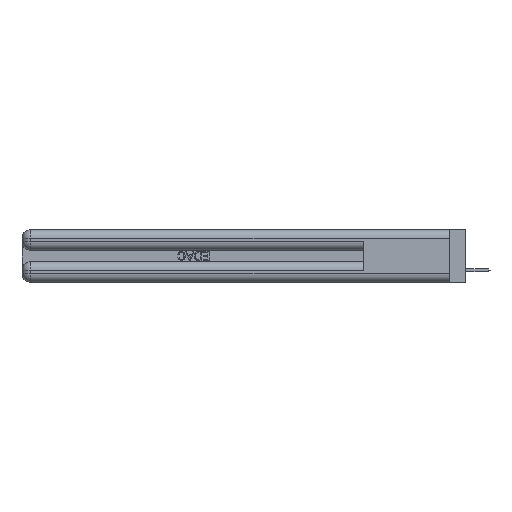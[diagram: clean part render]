
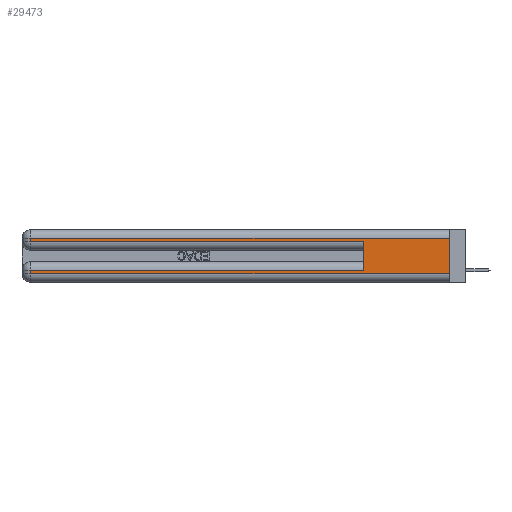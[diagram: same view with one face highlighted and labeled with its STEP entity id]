
A CAD part, left-side view. The second image highlights one B-rep face of the part: STEP entity #29473.
In plain terms, the highlighted planar face has unit normal (-1, 0, 0).
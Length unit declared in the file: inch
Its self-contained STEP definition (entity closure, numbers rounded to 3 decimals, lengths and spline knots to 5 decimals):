
#1678 = PLANE ( 'NONE',  #23824 ) ;
#2035 = CARTESIAN_POINT ( 'NONE',  ( 0., 0., 0.31 ) ) ;
#2815 = EDGE_CURVE ( 'NONE', #29592, #18097, #33552, .T. ) ;
#3059 = CARTESIAN_POINT ( 'NONE',  ( 0., 0.6, 0.285 ) ) ;
#4237 = ORIENTED_EDGE ( 'NONE', *, *, #30283, .T. ) ;
#4656 = VECTOR ( 'NONE', #31799, 39.37008 ) ;
#4960 = VERTEX_POINT ( 'NONE', #3059 ) ;
#5040 = DIRECTION ( 'NONE',  ( 0., -1., 0. ) ) ;
#5114 = EDGE_CURVE ( 'NONE', #21061, #26830, #23072, .T. ) ;
#5271 = VERTEX_POINT ( 'NONE', #16664 ) ;
#5775 = VECTOR ( 'NONE', #34278, 39.37008 ) ;
#7591 = DIRECTION ( 'NONE',  ( 0., 0., -1. ) ) ;
#9409 = EDGE_CURVE ( 'NONE', #21061, #18097, #37998, .T. ) ;
#9584 = ORIENTED_EDGE ( 'NONE', *, *, #9409, .F. ) ;
#10460 = CARTESIAN_POINT ( 'NONE',  ( 0., 0., 0.06 ) ) ;
#11641 = DIRECTION ( 'NONE',  ( 0., 1., 0. ) ) ;
#11681 = VECTOR ( 'NONE', #38478, 39.37008 ) ;
#12426 = VECTOR ( 'NONE', #5040, 39.37008 ) ;
#13044 = VERTEX_POINT ( 'NONE', #36705 ) ;
#13170 = CARTESIAN_POINT ( 'NONE',  ( 0., 2.94, 0.37 ) ) ;
#13666 = CARTESIAN_POINT ( 'NONE',  ( 0., 0., 0.37 ) ) ;
#13672 = CARTESIAN_POINT ( 'NONE',  ( 0., 2.94, 0.06 ) ) ;
#13814 = CARTESIAN_POINT ( 'NONE',  ( 0., 2.94, 0.31 ) ) ;
#14332 = VERTEX_POINT ( 'NONE', #25507 ) ;
#15169 = LINE ( 'NONE', #13170, #20305 ) ;
#15194 = CARTESIAN_POINT ( 'NONE',  ( 0., 0., 0.085 ) ) ;
#15325 = LINE ( 'NONE', #15194, #38266 ) ;
#16664 = CARTESIAN_POINT ( 'NONE',  ( 0., 2.94, 0.285 ) ) ;
#16717 = EDGE_LOOP ( 'NONE', ( #9584, #20422, #17849, #32713, #34236, #4237, #25037, #28146 ) ) ;
#17849 = ORIENTED_EDGE ( 'NONE', *, *, #28893, .T. ) ;
#18039 = CARTESIAN_POINT ( 'NONE',  ( 0., 0., 0.31 ) ) ;
#18097 = VERTEX_POINT ( 'NONE', #26007 ) ;
#19393 = CARTESIAN_POINT ( 'NONE',  ( 0., 0., 0.285 ) ) ;
#19431 = LINE ( 'NONE', #23124, #5775 ) ;
#20305 = VECTOR ( 'NONE', #28585, 39.37008 ) ;
#20422 = ORIENTED_EDGE ( 'NONE', *, *, #5114, .T. ) ;
#21035 = EDGE_CURVE ( 'NONE', #13044, #4960, #29566, .T. ) ;
#21061 = VERTEX_POINT ( 'NONE', #18039 ) ;
#22375 = DIRECTION ( 'NONE',  ( 0., -1., 0. ) ) ;
#22612 = FACE_OUTER_BOUND ( 'NONE', #16717, .T. ) ;
#23072 = LINE ( 'NONE', #2035, #29580 ) ;
#23124 = CARTESIAN_POINT ( 'NONE',  ( 0., 2.94, 0.37 ) ) ;
#23824 = AXIS2_PLACEMENT_3D ( 'NONE', #25743, #34540, #7591 ) ;
#25037 = ORIENTED_EDGE ( 'NONE', *, *, #27655, .T. ) ;
#25078 = VECTOR ( 'NONE', #22375, 39.37008 ) ;
#25507 = CARTESIAN_POINT ( 'NONE',  ( 0., 2.94, 0.085 ) ) ;
#25743 = CARTESIAN_POINT ( 'NONE',  ( 0., 0., 0.37 ) ) ;
#26007 = CARTESIAN_POINT ( 'NONE',  ( 0., 0., 0.06 ) ) ;
#26830 = VERTEX_POINT ( 'NONE', #13814 ) ;
#26874 = DIRECTION ( 'NONE',  ( 0., 1., 0. ) ) ;
#27184 = EDGE_CURVE ( 'NONE', #5271, #4960, #33089, .T. ) ;
#27655 = EDGE_CURVE ( 'NONE', #14332, #29592, #19431, .T. ) ;
#28146 = ORIENTED_EDGE ( 'NONE', *, *, #2815, .T. ) ;
#28585 = DIRECTION ( 'NONE',  ( 0., 0., -1. ) ) ;
#28893 = EDGE_CURVE ( 'NONE', #26830, #5271, #15169, .T. ) ;
#29473 = ADVANCED_FACE ( 'NONE', ( #22612 ), #1678, .F. ) ;
#29566 = LINE ( 'NONE', #34484, #11681 ) ;
#29580 = VECTOR ( 'NONE', #26874, 39.37008 ) ;
#29592 = VERTEX_POINT ( 'NONE', #13672 ) ;
#30283 = EDGE_CURVE ( 'NONE', #13044, #14332, #15325, .T. ) ;
#31799 = DIRECTION ( 'NONE',  ( 0., 0., -1. ) ) ;
#32713 = ORIENTED_EDGE ( 'NONE', *, *, #27184, .T. ) ;
#33089 = LINE ( 'NONE', #19393, #25078 ) ;
#33552 = LINE ( 'NONE', #10460, #12426 ) ;
#34236 = ORIENTED_EDGE ( 'NONE', *, *, #21035, .F. ) ;
#34278 = DIRECTION ( 'NONE',  ( 0., 0., -1. ) ) ;
#34484 = CARTESIAN_POINT ( 'NONE',  ( 0., 0.6, 0.145 ) ) ;
#34540 = DIRECTION ( 'NONE',  ( 1., 0., 0. ) ) ;
#36705 = CARTESIAN_POINT ( 'NONE',  ( 0., 0.6, 0.085 ) ) ;
#37998 = LINE ( 'NONE', #13666, #4656 ) ;
#38266 = VECTOR ( 'NONE', #11641, 39.37008 ) ;
#38478 = DIRECTION ( 'NONE',  ( 0., 0., 1. ) ) ;
